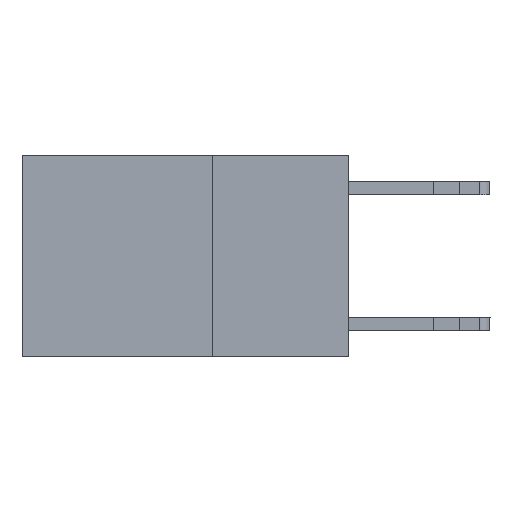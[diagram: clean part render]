
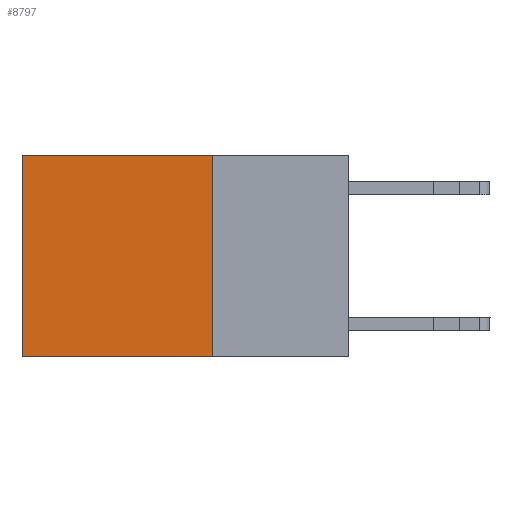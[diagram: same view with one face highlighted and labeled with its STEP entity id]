
A CAD part, left-side view. The second image highlights one B-rep face of the part: STEP entity #8797.
In plain terms, the highlighted planar face has unit normal (-1, 0, 0).
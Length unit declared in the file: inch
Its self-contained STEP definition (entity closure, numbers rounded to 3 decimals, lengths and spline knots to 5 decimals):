
#151 = AXIS2_PLACEMENT_3D ( 'NONE', #12068, #1344, #8208 ) ;
#769 = ORIENTED_EDGE ( 'NONE', *, *, #6376, .T. ) ;
#787 = VERTEX_POINT ( 'NONE', #2586 ) ;
#940 = CARTESIAN_POINT ( 'NONE',  ( 0.2625, 0.25, -0.37 ) ) ;
#978 = VECTOR ( 'NONE', #12660, 39.37008 ) ;
#1155 = LINE ( 'NONE', #1679, #8675 ) ;
#1344 = DIRECTION ( 'NONE',  ( 1., 0., 0. ) ) ;
#1611 = CARTESIAN_POINT ( 'NONE',  ( 0.2625, 0.6, 0. ) ) ;
#1679 = CARTESIAN_POINT ( 'NONE',  ( 0.2625, 0.25, 0. ) ) ;
#2283 = LINE ( 'NONE', #11952, #6842 ) ;
#2586 = CARTESIAN_POINT ( 'NONE',  ( 0.2625, 0.6, -0.37 ) ) ;
#3664 = LINE ( 'NONE', #940, #978 ) ;
#3678 = DIRECTION ( 'NONE',  ( 0., 1., 0. ) ) ;
#4032 = ORIENTED_EDGE ( 'NONE', *, *, #12233, .T. ) ;
#4270 = LINE ( 'NONE', #6305, #11689 ) ;
#4910 = FACE_OUTER_BOUND ( 'NONE', #7043, .T. ) ;
#6114 = DIRECTION ( 'NONE',  ( 0., 0., -1. ) ) ;
#6305 = CARTESIAN_POINT ( 'NONE',  ( 0.2625, 0.6, 0. ) ) ;
#6376 = EDGE_CURVE ( 'NONE', #8584, #7654, #1155, .T. ) ;
#6590 = EDGE_CURVE ( 'NONE', #12453, #787, #3664, .T. ) ;
#6842 = VECTOR ( 'NONE', #6114, 39.37008 ) ;
#7043 = EDGE_LOOP ( 'NONE', ( #4032, #11324, #11863, #769 ) ) ;
#7219 = PLANE ( 'NONE',  #151 ) ;
#7291 = DIRECTION ( 'NONE',  ( 0., 0., -1. ) ) ;
#7654 = VERTEX_POINT ( 'NONE', #1611 ) ;
#8208 = DIRECTION ( 'NONE',  ( 0., 0., -1. ) ) ;
#8584 = VERTEX_POINT ( 'NONE', #9820 ) ;
#8675 = VECTOR ( 'NONE', #3678, 39.37008 ) ;
#8797 = ADVANCED_FACE ( 'NONE', ( #4910 ), #7219, .F. ) ;
#9538 = CARTESIAN_POINT ( 'NONE',  ( 0.2625, 0.25, -0.37 ) ) ;
#9820 = CARTESIAN_POINT ( 'NONE',  ( 0.2625, 0.25, 0. ) ) ;
#10892 = EDGE_CURVE ( 'NONE', #8584, #12453, #2283, .T. ) ;
#11324 = ORIENTED_EDGE ( 'NONE', *, *, #6590, .F. ) ;
#11689 = VECTOR ( 'NONE', #7291, 39.37008 ) ;
#11863 = ORIENTED_EDGE ( 'NONE', *, *, #10892, .F. ) ;
#11952 = CARTESIAN_POINT ( 'NONE',  ( 0.2625, 0.25, 0. ) ) ;
#12068 = CARTESIAN_POINT ( 'NONE',  ( 0.2625, 0.25, 0. ) ) ;
#12233 = EDGE_CURVE ( 'NONE', #7654, #787, #4270, .T. ) ;
#12453 = VERTEX_POINT ( 'NONE', #9538 ) ;
#12660 = DIRECTION ( 'NONE',  ( 0., 1., 0. ) ) ;
